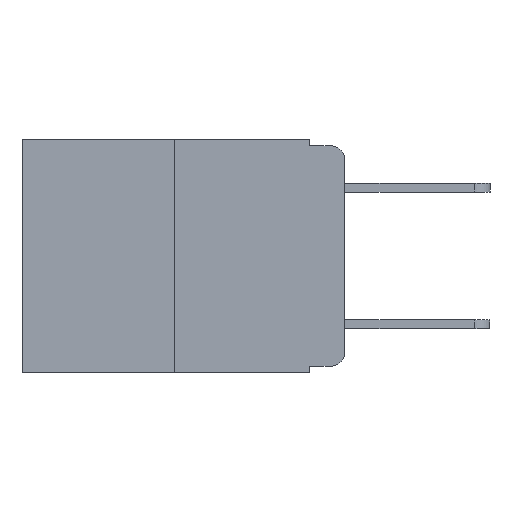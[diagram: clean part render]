
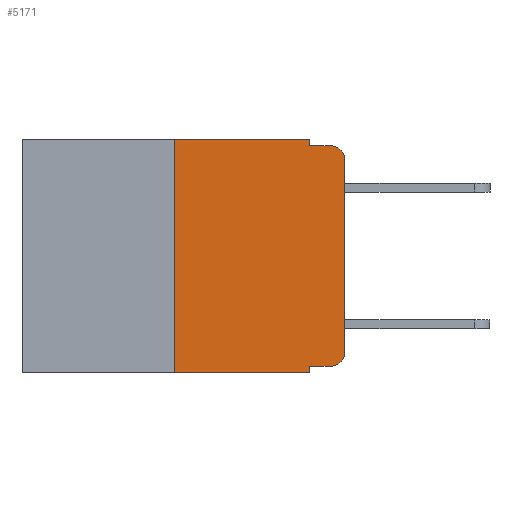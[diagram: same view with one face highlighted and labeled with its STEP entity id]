
A CAD part, left-side view. The second image highlights one B-rep face of the part: STEP entity #5171.
In plain terms, the highlighted planar face has unit normal (-1, 0, 0).
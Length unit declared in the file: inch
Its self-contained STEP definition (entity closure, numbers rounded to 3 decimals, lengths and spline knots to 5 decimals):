
#18 = PLANE ( 'NONE',  #1370 ) ;
#64 = CARTESIAN_POINT ( 'NONE',  ( 0., 0.02, -0.01 ) ) ;
#424 = CARTESIAN_POINT ( 'NONE',  ( 0., 0.051, 0. ) ) ;
#448 = CARTESIAN_POINT ( 'NONE',  ( 0., 0., -0.313 ) ) ;
#547 = EDGE_LOOP ( 'NONE', ( #5384, #7849, #4791, #1010, #10140, #7536, #8371, #1650, #7590, #1893 ) ) ;
#618 = VERTEX_POINT ( 'NONE', #4952 ) ;
#629 = VERTEX_POINT ( 'NONE', #8462 ) ;
#909 = CARTESIAN_POINT ( 'NONE',  ( 0., 0., 0. ) ) ;
#997 = VERTEX_POINT ( 'NONE', #1314 ) ;
#1003 = CARTESIAN_POINT ( 'NONE',  ( 0., 0.051, 0. ) ) ;
#1010 = ORIENTED_EDGE ( 'NONE', *, *, #5870, .F. ) ;
#1314 = CARTESIAN_POINT ( 'NONE',  ( 0., 0.051, -0.333 ) ) ;
#1320 = CARTESIAN_POINT ( 'NONE',  ( 0., 0.051, -0.01 ) ) ;
#1370 = AXIS2_PLACEMENT_3D ( 'NONE', #5529, #8475, #2243 ) ;
#1608 = AXIS2_PLACEMENT_3D ( 'NONE', #5601, #9345, #3331 ) ;
#1650 = ORIENTED_EDGE ( 'NONE', *, *, #5574, .F. ) ;
#1798 = DIRECTION ( 'NONE',  ( -1., 0., 0. ) ) ;
#1893 = ORIENTED_EDGE ( 'NONE', *, *, #4458, .T. ) ;
#2243 = DIRECTION ( 'NONE',  ( 0., 0., -1. ) ) ;
#2255 = VERTEX_POINT ( 'NONE', #64 ) ;
#2684 = CARTESIAN_POINT ( 'NONE',  ( 0., 0.25, 0. ) ) ;
#3197 = CARTESIAN_POINT ( 'NONE',  ( 0., 0.051, -0.333 ) ) ;
#3331 = DIRECTION ( 'NONE',  ( 0., 0., -1. ) ) ;
#3335 = CARTESIAN_POINT ( 'NONE',  ( 0., 0.02, -0.333 ) ) ;
#3337 = VECTOR ( 'NONE', #9110, 39.37008 ) ;
#3339 = DIRECTION ( 'NONE',  ( 0., 0., -1. ) ) ;
#3474 = VERTEX_POINT ( 'NONE', #10661 ) ;
#4015 = VECTOR ( 'NONE', #11841, 39.37008 ) ;
#4213 = VERTEX_POINT ( 'NONE', #6889 ) ;
#4416 = EDGE_CURVE ( 'NONE', #997, #7137, #11298, .T. ) ;
#4417 = VECTOR ( 'NONE', #10571, 39.37008 ) ;
#4458 = EDGE_CURVE ( 'NONE', #7137, #5955, #5680, .T. ) ;
#4602 = VERTEX_POINT ( 'NONE', #1320 ) ;
#4791 = ORIENTED_EDGE ( 'NONE', *, *, #5784, .F. ) ;
#4952 = CARTESIAN_POINT ( 'NONE',  ( 0., 0., -0.03 ) ) ;
#5171 = ADVANCED_FACE ( 'NONE', ( #7444 ), #18, .F. ) ;
#5201 = CARTESIAN_POINT ( 'NONE',  ( 0., 0.051, -0.01 ) ) ;
#5384 = ORIENTED_EDGE ( 'NONE', *, *, #5832, .T. ) ;
#5529 = CARTESIAN_POINT ( 'NONE',  ( 0., 0.473, 0. ) ) ;
#5574 = EDGE_CURVE ( 'NONE', #997, #629, #7175, .T. ) ;
#5592 = EDGE_CURVE ( 'NONE', #4213, #10015, #9039, .T. ) ;
#5601 = CARTESIAN_POINT ( 'NONE',  ( 0., 0.02, -0.313 ) ) ;
#5680 = CIRCLE ( 'NONE', #1608, 0.02 ) ;
#5763 = EDGE_CURVE ( 'NONE', #618, #2255, #7733, .T. ) ;
#5784 = EDGE_CURVE ( 'NONE', #4602, #2255, #11470, .T. ) ;
#5832 = EDGE_CURVE ( 'NONE', #5955, #618, #10819, .T. ) ;
#5870 = EDGE_CURVE ( 'NONE', #3474, #4602, #5972, .T. ) ;
#5955 = VERTEX_POINT ( 'NONE', #448 ) ;
#5972 = LINE ( 'NONE', #1003, #10391 ) ;
#6475 = EDGE_CURVE ( 'NONE', #10015, #3474, #9289, .T. ) ;
#6517 = DIRECTION ( 'NONE',  ( 0., -1., 0. ) ) ;
#6644 = VECTOR ( 'NONE', #6517, 39.37008 ) ;
#6684 = EDGE_CURVE ( 'NONE', #4213, #629, #10699, .T. ) ;
#6889 = CARTESIAN_POINT ( 'NONE',  ( 0., 0.25, -0.343 ) ) ;
#7085 = CARTESIAN_POINT ( 'NONE',  ( 0., 0.25, 0. ) ) ;
#7137 = VERTEX_POINT ( 'NONE', #3335 ) ;
#7175 = LINE ( 'NONE', #424, #9312 ) ;
#7444 = FACE_OUTER_BOUND ( 'NONE', #547, .T. ) ;
#7536 = ORIENTED_EDGE ( 'NONE', *, *, #5592, .F. ) ;
#7590 = ORIENTED_EDGE ( 'NONE', *, *, #4416, .T. ) ;
#7733 = CIRCLE ( 'NONE', #9729, 0.02 ) ;
#7849 = ORIENTED_EDGE ( 'NONE', *, *, #5763, .T. ) ;
#8036 = CARTESIAN_POINT ( 'NONE',  ( 0., 0.02, -0.03 ) ) ;
#8322 = VECTOR ( 'NONE', #9267, 39.37008 ) ;
#8371 = ORIENTED_EDGE ( 'NONE', *, *, #6684, .T. ) ;
#8402 = CARTESIAN_POINT ( 'NONE',  ( 0., 0.473, -0.343 ) ) ;
#8462 = CARTESIAN_POINT ( 'NONE',  ( 0., 0.051, -0.343 ) ) ;
#8475 = DIRECTION ( 'NONE',  ( 1., 0., 0. ) ) ;
#8785 = VECTOR ( 'NONE', #11101, 39.37008 ) ;
#8965 = DIRECTION ( 'NONE',  ( 0., 0., -1. ) ) ;
#9039 = LINE ( 'NONE', #2684, #8785 ) ;
#9110 = DIRECTION ( 'NONE',  ( 0., 0., 1. ) ) ;
#9267 = DIRECTION ( 'NONE',  ( 0., -1., 0. ) ) ;
#9289 = LINE ( 'NONE', #9737, #4015 ) ;
#9312 = VECTOR ( 'NONE', #11725, 39.37008 ) ;
#9345 = DIRECTION ( 'NONE',  ( -1., 0., 0. ) ) ;
#9729 = AXIS2_PLACEMENT_3D ( 'NONE', #8036, #1798, #8965 ) ;
#9737 = CARTESIAN_POINT ( 'NONE',  ( 0., 0.473, 0. ) ) ;
#10015 = VERTEX_POINT ( 'NONE', #7085 ) ;
#10140 = ORIENTED_EDGE ( 'NONE', *, *, #6475, .F. ) ;
#10391 = VECTOR ( 'NONE', #3339, 39.37008 ) ;
#10571 = DIRECTION ( 'NONE',  ( 0., -1., 0. ) ) ;
#10661 = CARTESIAN_POINT ( 'NONE',  ( 0., 0.051, 0. ) ) ;
#10699 = LINE ( 'NONE', #8402, #8322 ) ;
#10819 = LINE ( 'NONE', #909, #3337 ) ;
#11101 = DIRECTION ( 'NONE',  ( 0., 0., 1. ) ) ;
#11298 = LINE ( 'NONE', #3197, #6644 ) ;
#11470 = LINE ( 'NONE', #5201, #4417 ) ;
#11725 = DIRECTION ( 'NONE',  ( 0., 0., -1. ) ) ;
#11841 = DIRECTION ( 'NONE',  ( 0., -1., 0. ) ) ;
